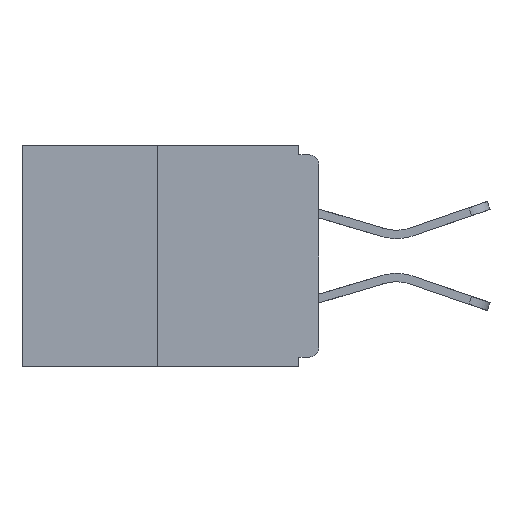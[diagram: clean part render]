
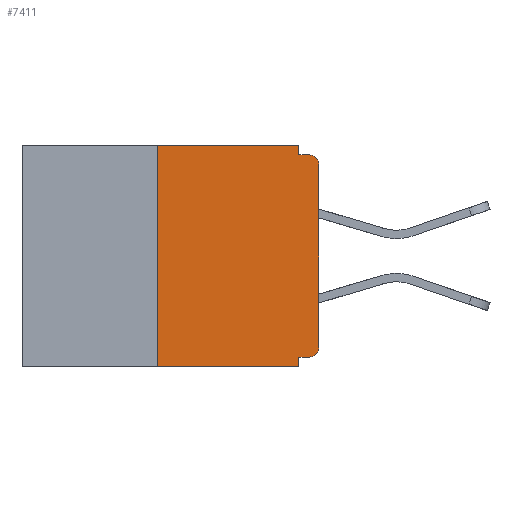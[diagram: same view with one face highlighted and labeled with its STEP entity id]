
A CAD part, left-side view. The second image highlights one B-rep face of the part: STEP entity #7411.
In plain terms, the highlighted planar face has unit normal (-1, 0, 0).
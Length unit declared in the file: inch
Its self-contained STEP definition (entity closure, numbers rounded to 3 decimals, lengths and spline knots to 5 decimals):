
#17 = DIRECTION ( 'NONE',  ( 0., -1., 0. ) ) ;
#934 = ORIENTED_EDGE ( 'NONE', *, *, #5454, .F. ) ;
#998 = EDGE_CURVE ( 'NONE', #2505, #5992, #15736, .T. ) ;
#1058 = CARTESIAN_POINT ( 'NONE',  ( 0., 0.015, -0.313 ) ) ;
#1323 = CARTESIAN_POINT ( 'NONE',  ( 0., 0.015, -0.328 ) ) ;
#1333 = CARTESIAN_POINT ( 'NONE',  ( 0., 0.25, 0. ) ) ;
#1343 = LINE ( 'NONE', #6879, #12178 ) ;
#1597 = EDGE_CURVE ( 'NONE', #10923, #3020, #10005, .T. ) ;
#1617 = EDGE_CURVE ( 'NONE', #14423, #13698, #14362, .T. ) ;
#2168 = PLANE ( 'NONE',  #3998 ) ;
#2403 = VERTEX_POINT ( 'NONE', #12634 ) ;
#2505 = VERTEX_POINT ( 'NONE', #14060 ) ;
#2611 = CARTESIAN_POINT ( 'NONE',  ( 0., 0.031, -0.343 ) ) ;
#2766 = VECTOR ( 'NONE', #5805, 39.37008 ) ;
#3020 = VERTEX_POINT ( 'NONE', #12302 ) ;
#3386 = CARTESIAN_POINT ( 'NONE',  ( 0., 0.46, 0. ) ) ;
#3495 = CIRCLE ( 'NONE', #4315, 0.015 ) ;
#3998 = AXIS2_PLACEMENT_3D ( 'NONE', #3386, #8293, #9402 ) ;
#4179 = LINE ( 'NONE', #1333, #10621 ) ;
#4289 = EDGE_CURVE ( 'NONE', #6579, #2505, #1343, .T. ) ;
#4315 = AXIS2_PLACEMENT_3D ( 'NONE', #1058, #9595, #14456 ) ;
#4710 = VECTOR ( 'NONE', #17, 39.37008 ) ;
#4903 = CARTESIAN_POINT ( 'NONE',  ( 0., 0.015, -0.03 ) ) ;
#4923 = CARTESIAN_POINT ( 'NONE',  ( 0., 0.031, -0.343 ) ) ;
#5454 = EDGE_CURVE ( 'NONE', #14423, #10643, #4179, .T. ) ;
#5492 = CARTESIAN_POINT ( 'NONE',  ( 0., 0.25, -0.343 ) ) ;
#5587 = ORIENTED_EDGE ( 'NONE', *, *, #4289, .F. ) ;
#5611 = ORIENTED_EDGE ( 'NONE', *, *, #13228, .F. ) ;
#5791 = CARTESIAN_POINT ( 'NONE',  ( 0., 0.25, 0. ) ) ;
#5805 = DIRECTION ( 'NONE',  ( 0., 1., 0. ) ) ;
#5809 = VERTEX_POINT ( 'NONE', #11185 ) ;
#5992 = VERTEX_POINT ( 'NONE', #12930 ) ;
#6026 = DIRECTION ( 'NONE',  ( 0., 0., -1. ) ) ;
#6448 = ORIENTED_EDGE ( 'NONE', *, *, #998, .F. ) ;
#6579 = VERTEX_POINT ( 'NONE', #14802 ) ;
#6865 = VECTOR ( 'NONE', #15275, 39.37008 ) ;
#6879 = CARTESIAN_POINT ( 'NONE',  ( 0., 0.031, 0. ) ) ;
#7231 = CARTESIAN_POINT ( 'NONE',  ( 0., 0.46, -0.343 ) ) ;
#7259 = LINE ( 'NONE', #4923, #10092 ) ;
#7411 = ADVANCED_FACE ( 'NONE', ( #9017 ), #2168, .F. ) ;
#8065 = EDGE_CURVE ( 'NONE', #10923, #2403, #3495, .T. ) ;
#8117 = CARTESIAN_POINT ( 'NONE',  ( 0., 0., -0.015 ) ) ;
#8224 = CARTESIAN_POINT ( 'NONE',  ( 0., 0., 0. ) ) ;
#8241 = CIRCLE ( 'NONE', #9303, 0.015 ) ;
#8286 = EDGE_CURVE ( 'NONE', #5809, #5992, #8241, .T. ) ;
#8293 = DIRECTION ( 'NONE',  ( 1., 0., 0. ) ) ;
#8492 = ORIENTED_EDGE ( 'NONE', *, *, #11126, .T. ) ;
#9017 = FACE_OUTER_BOUND ( 'NONE', #10502, .T. ) ;
#9303 = AXIS2_PLACEMENT_3D ( 'NONE', #4903, #14473, #6026 ) ;
#9402 = DIRECTION ( 'NONE',  ( 0., 0., -1. ) ) ;
#9595 = DIRECTION ( 'NONE',  ( -1., 0., 0. ) ) ;
#9844 = DIRECTION ( 'NONE',  ( 0., 0., 1. ) ) ;
#10005 = LINE ( 'NONE', #14950, #2766 ) ;
#10063 = ORIENTED_EDGE ( 'NONE', *, *, #1597, .F. ) ;
#10092 = VECTOR ( 'NONE', #14649, 39.37008 ) ;
#10502 = EDGE_LOOP ( 'NONE', ( #5611, #934, #11925, #12436, #10063, #15635, #8492, #13000, #6448, #5587 ) ) ;
#10621 = VECTOR ( 'NONE', #9844, 39.37008 ) ;
#10643 = VERTEX_POINT ( 'NONE', #5791 ) ;
#10923 = VERTEX_POINT ( 'NONE', #1323 ) ;
#11126 = EDGE_CURVE ( 'NONE', #2403, #5809, #14984, .T. ) ;
#11185 = CARTESIAN_POINT ( 'NONE',  ( 0., 0., -0.03 ) ) ;
#11384 = CARTESIAN_POINT ( 'NONE',  ( 0., 0.46, 0. ) ) ;
#11680 = DIRECTION ( 'NONE',  ( 0., 0., -1. ) ) ;
#11925 = ORIENTED_EDGE ( 'NONE', *, *, #1617, .T. ) ;
#12178 = VECTOR ( 'NONE', #11680, 39.37008 ) ;
#12212 = VECTOR ( 'NONE', #12760, 39.37008 ) ;
#12302 = CARTESIAN_POINT ( 'NONE',  ( 0., 0.031, -0.328 ) ) ;
#12436 = ORIENTED_EDGE ( 'NONE', *, *, #14165, .F. ) ;
#12487 = VECTOR ( 'NONE', #14095, 39.37008 ) ;
#12634 = CARTESIAN_POINT ( 'NONE',  ( 0., 0., -0.313 ) ) ;
#12760 = DIRECTION ( 'NONE',  ( 0., -1., 0. ) ) ;
#12774 = LINE ( 'NONE', #11384, #12212 ) ;
#12930 = CARTESIAN_POINT ( 'NONE',  ( 0., 0.015, -0.015 ) ) ;
#13000 = ORIENTED_EDGE ( 'NONE', *, *, #8286, .T. ) ;
#13228 = EDGE_CURVE ( 'NONE', #10643, #6579, #12774, .T. ) ;
#13698 = VERTEX_POINT ( 'NONE', #2611 ) ;
#14060 = CARTESIAN_POINT ( 'NONE',  ( 0., 0.031, -0.015 ) ) ;
#14095 = DIRECTION ( 'NONE',  ( 0., -1., 0. ) ) ;
#14165 = EDGE_CURVE ( 'NONE', #3020, #13698, #7259, .T. ) ;
#14362 = LINE ( 'NONE', #7231, #4710 ) ;
#14423 = VERTEX_POINT ( 'NONE', #5492 ) ;
#14456 = DIRECTION ( 'NONE',  ( 0., 0., -1. ) ) ;
#14473 = DIRECTION ( 'NONE',  ( -1., 0., 0. ) ) ;
#14649 = DIRECTION ( 'NONE',  ( 0., 0., -1. ) ) ;
#14802 = CARTESIAN_POINT ( 'NONE',  ( 0., 0.031, 0. ) ) ;
#14950 = CARTESIAN_POINT ( 'NONE',  ( 0., 0., -0.328 ) ) ;
#14984 = LINE ( 'NONE', #8224, #6865 ) ;
#15275 = DIRECTION ( 'NONE',  ( 0., 0., 1. ) ) ;
#15635 = ORIENTED_EDGE ( 'NONE', *, *, #8065, .T. ) ;
#15736 = LINE ( 'NONE', #8117, #12487 ) ;
